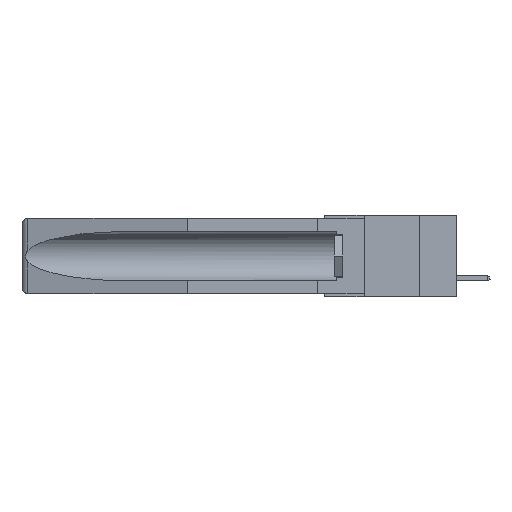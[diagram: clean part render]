
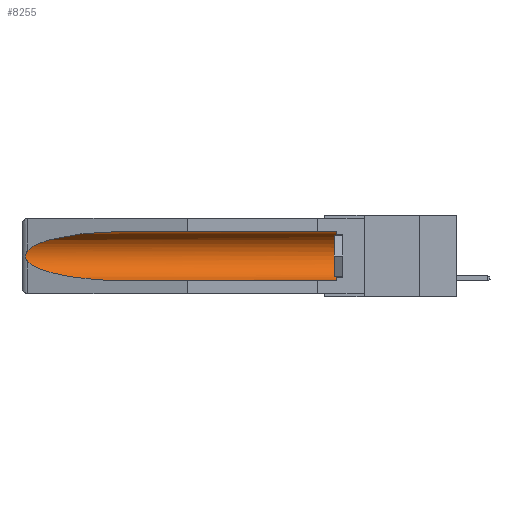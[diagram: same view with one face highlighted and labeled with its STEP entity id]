
A CAD part, left-side view. The second image highlights one B-rep face of the part: STEP entity #8255.
In plain terms, the highlighted cylindrical face has radius 2.857 mm (diameter 5.715 mm), a partial arc.
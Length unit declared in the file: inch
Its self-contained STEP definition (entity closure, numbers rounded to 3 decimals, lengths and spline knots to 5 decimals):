
#127 = CARTESIAN_POINT ( 'NONE',  ( 0.155, -0.30754, -0.1715 ) ) ;
#592 = CARTESIAN_POINT ( 'NONE',  ( 0.26537, 1.52718, -0.14972 ) ) ;
#645 = LINE ( 'NONE', #9088, #17584 ) ;
#1815 = EDGE_CURVE ( 'NONE', #17477, #19791, #12656, .T. ) ;
#2112 = CARTESIAN_POINT ( 'NONE',  ( 0.26537, 1.52718, -0.19328 ) ) ;
#2652 = ORIENTED_EDGE ( 'NONE', *, *, #12395, .T. ) ;
#2851 = LINE ( 'NONE', #19779, #6305 ) ;
#2943 = CARTESIAN_POINT ( 'NONE',  ( 0.2673, 1.5327, -0.16383 ) ) ;
#3199 = DIRECTION ( 'NONE',  ( 0., 1., 0. ) ) ;
#3213 = CARTESIAN_POINT ( 'NONE',  ( 0.2673, 1.53269, -0.17917 ) ) ;
#3537 = CARTESIAN_POINT ( 'NONE',  ( 0.26537, 1.52718, -0.14972 ) ) ;
#3545 = CARTESIAN_POINT ( 'NONE',  ( 0.26537, 1.52718, -0.19328 ) ) ;
#3789 = CARTESIAN_POINT ( 'NONE',  ( 0.155, 1.07973, -0.284 ) ) ;
#4099 = CARTESIAN_POINT ( 'NONE',  ( 0.155, 0.126, -0.1715 ) ) ;
#4812 = CARTESIAN_POINT ( 'NONE',  ( 0.26597, 1.5296, -0.19026 ) ) ;
#5087 =( BOUNDED_CURVE ( )  B_SPLINE_CURVE ( 3, ( #9979, #6757, #8124, #592 ),
 .UNSPECIFIED., .F., .F. ) 
 B_SPLINE_CURVE_WITH_KNOTS ( ( 4, 4 ),
 ( 4.71239, 6.08839 ),
 .UNSPECIFIED. ) 
 CURVE ( )  GEOMETRIC_REPRESENTATION_ITEM ( )  RATIONAL_B_SPLINE_CURVE ( ( 1., 0.848, 0.848, 1. ) ) 
 REPRESENTATION_ITEM ( '' )  );
#5432 = EDGE_CURVE ( 'NONE', #12379, #17328, #6563, .T. ) ;
#5718 = DIRECTION ( 'NONE',  ( 0., 1., 0. ) ) ;
#5972 = VERTEX_POINT ( 'NONE', #6692 ) ;
#6305 = VECTOR ( 'NONE', #5718, 39.37008 ) ;
#6474 = EDGE_CURVE ( 'NONE', #19791, #5972, #645, .T. ) ;
#6563 = B_SPLINE_CURVE_WITH_KNOTS ( 'NONE', 3,
 ( #12466, #9450, #15702, #2943, #13906, #9380, #3213, #14192, #4812, #3545 ),
 .UNSPECIFIED., .F., .F.,
 ( 4, 2, 2, 2, 4 ),
 ( 0., 0.00029, 0.00058, 0.00087, 0.00117 ),
 .UNSPECIFIED. ) ;
#6692 = CARTESIAN_POINT ( 'NONE',  ( 0.155, 1.07973, -0.059 ) ) ;
#6757 = CARTESIAN_POINT ( 'NONE',  ( 0.21114, 1.30732, -0.059 ) ) ;
#7381 = CYLINDRICAL_SURFACE ( 'NONE', #7824, 0.1125 ) ;
#7824 = AXIS2_PLACEMENT_3D ( 'NONE', #127, #3199, #19258 ) ;
#8124 = CARTESIAN_POINT ( 'NONE',  ( 0.25451, 1.48313, -0.09465 ) ) ;
#8255 = ADVANCED_FACE ( 'NONE', ( #15600 ), #7381, .F. ) ;
#9088 = CARTESIAN_POINT ( 'NONE',  ( 0.155, -0.30754, -0.059 ) ) ;
#9154 = DIRECTION ( 'NONE',  ( 0., 0., 1. ) ) ;
#9380 = CARTESIAN_POINT ( 'NONE',  ( 0.2675, 1.53308, -0.17534 ) ) ;
#9450 = CARTESIAN_POINT ( 'NONE',  ( 0.26597, 1.52961, -0.15275 ) ) ;
#9926 = CARTESIAN_POINT ( 'NONE',  ( 0.155, 1.07973, -0.284 ) ) ;
#9979 = CARTESIAN_POINT ( 'NONE',  ( 0.155, 1.07973, -0.059 ) ) ;
#9982 = CARTESIAN_POINT ( 'NONE',  ( 0.21114, 1.30732, -0.284 ) ) ;
#10798 = EDGE_CURVE ( 'NONE', #17477, #14492, #2851, .T. ) ;
#11434 = CARTESIAN_POINT ( 'NONE',  ( 0.25451, 1.48313, -0.24835 ) ) ;
#11571 = CARTESIAN_POINT ( 'NONE',  ( 0.155, 0.126, -0.284 ) ) ;
#12379 = VERTEX_POINT ( 'NONE', #3537 ) ;
#12395 = EDGE_CURVE ( 'NONE', #5972, #12379, #5087, .T. ) ;
#12466 = CARTESIAN_POINT ( 'NONE',  ( 0.26537, 1.52718, -0.14972 ) ) ;
#12656 = CIRCLE ( 'NONE', #13543, 0.1125 ) ;
#13543 = AXIS2_PLACEMENT_3D ( 'NONE', #4099, #16664, #9154 ) ;
#13688 = DIRECTION ( 'NONE',  ( 0., 1., 0. ) ) ;
#13906 = CARTESIAN_POINT ( 'NONE',  ( 0.2675, 1.53308, -0.16763 ) ) ;
#14182 = EDGE_CURVE ( 'NONE', #17328, #14492, #16633, .T. ) ;
#14192 = CARTESIAN_POINT ( 'NONE',  ( 0.26655, 1.53094, -0.18657 ) ) ;
#14492 = VERTEX_POINT ( 'NONE', #3789 ) ;
#14772 = ORIENTED_EDGE ( 'NONE', *, *, #1815, .T. ) ;
#15600 = FACE_OUTER_BOUND ( 'NONE', #19671, .T. ) ;
#15702 = CARTESIAN_POINT ( 'NONE',  ( 0.26654, 1.53092, -0.15636 ) ) ;
#15974 = ORIENTED_EDGE ( 'NONE', *, *, #14182, .T. ) ;
#16633 =( BOUNDED_CURVE ( )  B_SPLINE_CURVE ( 3, ( #2112, #11434, #9982, #9926 ),
 .UNSPECIFIED., .F., .F. ) 
 B_SPLINE_CURVE_WITH_KNOTS ( ( 4, 4 ),
 ( 0.1948, 1.5708 ),
 .UNSPECIFIED. ) 
 CURVE ( )  GEOMETRIC_REPRESENTATION_ITEM ( )  RATIONAL_B_SPLINE_CURVE ( ( 1., 0.848, 0.848, 1. ) ) 
 REPRESENTATION_ITEM ( '' )  );
#16664 = DIRECTION ( 'NONE',  ( 0., -1., 0. ) ) ;
#16806 = ORIENTED_EDGE ( 'NONE', *, *, #5432, .T. ) ;
#17270 = ORIENTED_EDGE ( 'NONE', *, *, #6474, .T. ) ;
#17328 = VERTEX_POINT ( 'NONE', #18991 ) ;
#17477 = VERTEX_POINT ( 'NONE', #11571 ) ;
#17584 = VECTOR ( 'NONE', #13688, 39.37008 ) ;
#17901 = ORIENTED_EDGE ( 'NONE', *, *, #10798, .F. ) ;
#18991 = CARTESIAN_POINT ( 'NONE',  ( 0.26537, 1.52718, -0.19328 ) ) ;
#19258 = DIRECTION ( 'NONE',  ( 0., 0., 1. ) ) ;
#19671 = EDGE_LOOP ( 'NONE', ( #2652, #16806, #15974, #17901, #14772, #17270 ) ) ;
#19779 = CARTESIAN_POINT ( 'NONE',  ( 0.155, -0.30754, -0.284 ) ) ;
#19791 = VERTEX_POINT ( 'NONE', #20324 ) ;
#20324 = CARTESIAN_POINT ( 'NONE',  ( 0.155, 0.126, -0.059 ) ) ;
